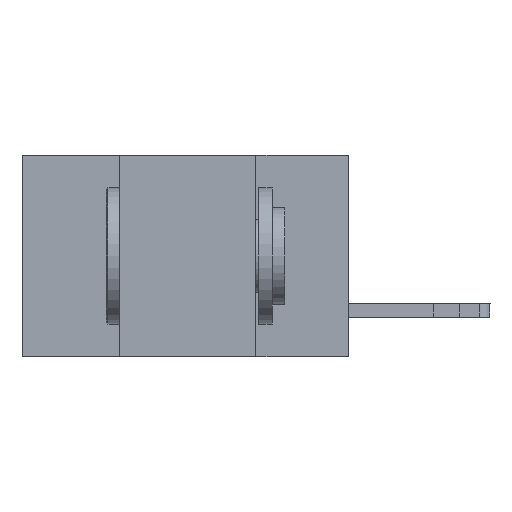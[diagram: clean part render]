
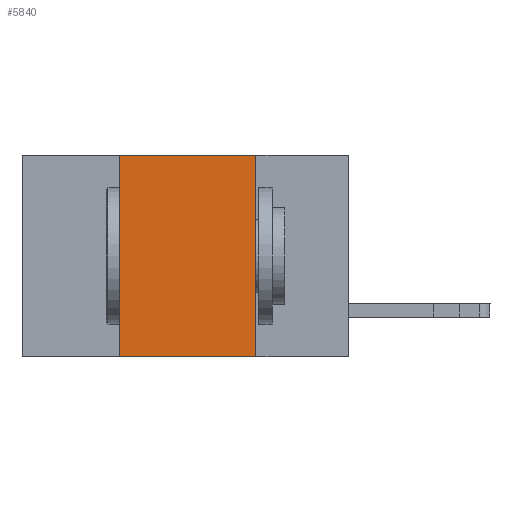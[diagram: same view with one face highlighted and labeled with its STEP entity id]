
A CAD part, left-side view. The second image highlights one B-rep face of the part: STEP entity #5840.
In plain terms, the highlighted planar face has unit normal (-1, 0, 0).
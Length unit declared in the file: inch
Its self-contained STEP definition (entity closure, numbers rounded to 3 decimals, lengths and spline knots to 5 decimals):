
#1312 = CARTESIAN_POINT ( 'NONE',  ( 0., 0.17, 0. ) ) ;
#1710 = CARTESIAN_POINT ( 'NONE',  ( 0., 0.42, 0. ) ) ;
#2298 = VERTEX_POINT ( 'NONE', #1710 ) ;
#2728 = VECTOR ( 'NONE', #12785, 39.37008 ) ;
#2848 = EDGE_CURVE ( 'NONE', #5119, #9916, #13447, .T. ) ;
#2898 = VECTOR ( 'NONE', #9461, 39.37008 ) ;
#3784 = ORIENTED_EDGE ( 'NONE', *, *, #2848, .T. ) ;
#3881 = VECTOR ( 'NONE', #4335, 39.37008 ) ;
#4335 = DIRECTION ( 'NONE',  ( 0., 0., -1. ) ) ;
#5119 = VERTEX_POINT ( 'NONE', #12214 ) ;
#5451 = ORIENTED_EDGE ( 'NONE', *, *, #8610, .F. ) ;
#5840 = ADVANCED_FACE ( 'NONE', ( #10032 ), #13300, .F. ) ;
#7178 = VECTOR ( 'NONE', #9337, 39.37008 ) ;
#7210 = EDGE_LOOP ( 'NONE', ( #11039, #11684, #5451, #3784 ) ) ;
#7596 = EDGE_CURVE ( 'NONE', #2298, #13841, #10067, .T. ) ;
#8382 = CARTESIAN_POINT ( 'NONE',  ( 0., 0.42, -0.37 ) ) ;
#8610 = EDGE_CURVE ( 'NONE', #5119, #2298, #11485, .T. ) ;
#9337 = DIRECTION ( 'NONE',  ( 0., -1., 0. ) ) ;
#9461 = DIRECTION ( 'NONE',  ( 0., 0., 1. ) ) ;
#9526 = CARTESIAN_POINT ( 'NONE',  ( 0., 0.6, 0. ) ) ;
#9916 = VERTEX_POINT ( 'NONE', #10200 ) ;
#10032 = FACE_OUTER_BOUND ( 'NONE', #7210, .T. ) ;
#10067 = LINE ( 'NONE', #9526, #7178 ) ;
#10200 = CARTESIAN_POINT ( 'NONE',  ( 0., 0.17, -0.37 ) ) ;
#11039 = ORIENTED_EDGE ( 'NONE', *, *, #12574, .F. ) ;
#11485 = LINE ( 'NONE', #8382, #2898 ) ;
#11684 = ORIENTED_EDGE ( 'NONE', *, *, #7596, .F. ) ;
#11877 = CARTESIAN_POINT ( 'NONE',  ( 0., 0.17, -0.37 ) ) ;
#12214 = CARTESIAN_POINT ( 'NONE',  ( 0., 0.42, -0.37 ) ) ;
#12454 = LINE ( 'NONE', #11877, #3881 ) ;
#12574 = EDGE_CURVE ( 'NONE', #13841, #9916, #12454, .T. ) ;
#12785 = DIRECTION ( 'NONE',  ( 0., -1., 0. ) ) ;
#12816 = CARTESIAN_POINT ( 'NONE',  ( 0., 0.6, -0.37 ) ) ;
#12864 = DIRECTION ( 'NONE',  ( 0., 0., -1. ) ) ;
#12917 = DIRECTION ( 'NONE',  ( 1., 0., 0. ) ) ;
#13209 = CARTESIAN_POINT ( 'NONE',  ( 0., 0.6, 0. ) ) ;
#13300 = PLANE ( 'NONE',  #13588 ) ;
#13447 = LINE ( 'NONE', #12816, #2728 ) ;
#13588 = AXIS2_PLACEMENT_3D ( 'NONE', #13209, #12917, #12864 ) ;
#13841 = VERTEX_POINT ( 'NONE', #1312 ) ;
